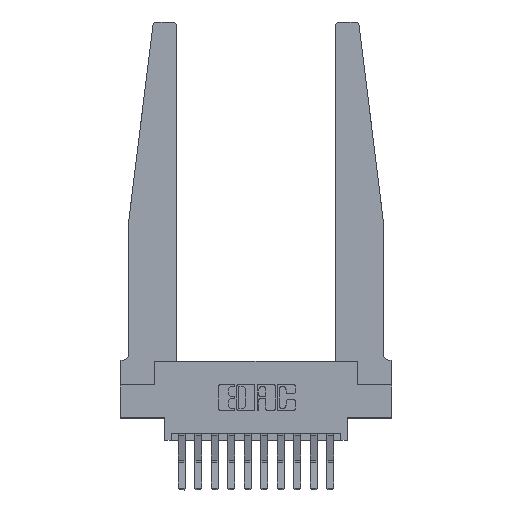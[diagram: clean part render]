
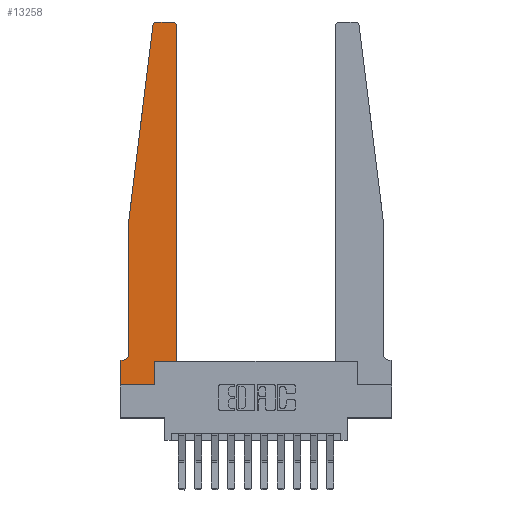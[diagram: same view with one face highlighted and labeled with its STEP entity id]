
A CAD part, top view. The second image highlights one B-rep face of the part: STEP entity #13258.
In plain terms, the highlighted planar face has unit normal (0, 0, 1).
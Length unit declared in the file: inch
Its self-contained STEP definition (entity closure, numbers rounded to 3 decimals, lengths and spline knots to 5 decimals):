
#75 = VERTEX_POINT ( 'NONE', #12826 ) ;
#86 = LINE ( 'NONE', #15667, #2582 ) ;
#128 = EDGE_CURVE ( 'NONE', #75, #3566, #86, .T. ) ;
#212 = DIRECTION ( 'NONE',  ( 0., 0., 1. ) ) ;
#662 = ORIENTED_EDGE ( 'NONE', *, *, #15537, .T. ) ;
#775 = AXIS2_PLACEMENT_3D ( 'NONE', #14170, #6856, #15410 ) ;
#1500 = LINE ( 'NONE', #12822, #10864 ) ;
#1690 = LINE ( 'NONE', #8300, #11048 ) ;
#1749 = EDGE_CURVE ( 'NONE', #13895, #6172, #13241, .T. ) ;
#2089 = EDGE_CURVE ( 'NONE', #12580, #13895, #5752, .T. ) ;
#2169 = DIRECTION ( 'NONE',  ( -0.122, -0.992, 0. ) ) ;
#2582 = VECTOR ( 'NONE', #8376, 39.37008 ) ;
#2801 = VERTEX_POINT ( 'NONE', #6228 ) ;
#3094 = VECTOR ( 'NONE', #2169, 39.37008 ) ;
#3345 = CARTESIAN_POINT ( 'NONE',  ( 0., 0.1875, 0.37 ) ) ;
#3473 = VECTOR ( 'NONE', #4188, 39.37008 ) ;
#3566 = VERTEX_POINT ( 'NONE', #9481 ) ;
#3702 = EDGE_CURVE ( 'NONE', #12538, #7731, #10699, .T. ) ;
#3711 = CARTESIAN_POINT ( 'NONE',  ( 0., 0.1875, 0.37 ) ) ;
#4159 = LINE ( 'NONE', #6285, #13909 ) ;
#4188 = DIRECTION ( 'NONE',  ( 1., 0., 0. ) ) ;
#4594 = DIRECTION ( 'NONE',  ( 0., 0., -1. ) ) ;
#4637 = DIRECTION ( 'NONE',  ( 0., -1., 0. ) ) ;
#4796 = CARTESIAN_POINT ( 'NONE',  ( 0., 0., 0.37 ) ) ;
#4827 = CARTESIAN_POINT ( 'NONE',  ( 0.2605, 0.18, 0.37 ) ) ;
#4869 = CARTESIAN_POINT ( 'NONE',  ( 0.425, 0.18, 0.37 ) ) ;
#5153 = EDGE_CURVE ( 'NONE', #2801, #8428, #14705, .T. ) ;
#5361 = CARTESIAN_POINT ( 'NONE',  ( 0.425, 0.18, 0.37 ) ) ;
#5443 = AXIS2_PLACEMENT_3D ( 'NONE', #3345, #7037, #15584 ) ;
#5482 = DIRECTION ( 'NONE',  ( -1., 0., 0. ) ) ;
#5547 = AXIS2_PLACEMENT_3D ( 'NONE', #7550, #212, #8792 ) ;
#5752 = LINE ( 'NONE', #4827, #11909 ) ;
#5829 = EDGE_LOOP ( 'NONE', ( #662, #6163, #9214, #6130, #12266, #8538, #13046, #6628, #7560, #15074, #10720, #9057 ) ) ;
#5873 = CARTESIAN_POINT ( 'NONE',  ( 0.015, 0.1875, 0.37 ) ) ;
#6130 = ORIENTED_EDGE ( 'NONE', *, *, #128, .T. ) ;
#6163 = ORIENTED_EDGE ( 'NONE', *, *, #3702, .T. ) ;
#6172 = VERTEX_POINT ( 'NONE', #4869 ) ;
#6228 = CARTESIAN_POINT ( 'NONE',  ( 0.425, 2.72, 0.37 ) ) ;
#6285 = CARTESIAN_POINT ( 'NONE',  ( 0., 0., 0.37 ) ) ;
#6332 = LINE ( 'NONE', #9475, #3094 ) ;
#6562 = CARTESIAN_POINT ( 'NONE',  ( 0.395, 2.75, 0.37 ) ) ;
#6628 = ORIENTED_EDGE ( 'NONE', *, *, #15398, .T. ) ;
#6856 = DIRECTION ( 'NONE',  ( 0., 0., 1. ) ) ;
#7037 = DIRECTION ( 'NONE',  ( 0., 0., 1. ) ) ;
#7222 = CARTESIAN_POINT ( 'NONE',  ( 0.065, 0.1875, 0.37 ) ) ;
#7550 = CARTESIAN_POINT ( 'NONE',  ( 0.27653, 2.72, 0.37 ) ) ;
#7560 = ORIENTED_EDGE ( 'NONE', *, *, #2089, .T. ) ;
#7731 = VERTEX_POINT ( 'NONE', #9168 ) ;
#8075 = EDGE_CURVE ( 'NONE', #12221, #10811, #9662, .T. ) ;
#8299 = DIRECTION ( 'NONE',  ( 0., 1., 0. ) ) ;
#8300 = CARTESIAN_POINT ( 'NONE',  ( 0., 0., 0.37 ) ) ;
#8320 = CIRCLE ( 'NONE', #14094, 0.05 ) ;
#8376 = DIRECTION ( 'NONE',  ( 0., -1., 0. ) ) ;
#8428 = VERTEX_POINT ( 'NONE', #6562 ) ;
#8532 = DIRECTION ( 'NONE',  ( 0., 1., 0. ) ) ;
#8538 = ORIENTED_EDGE ( 'NONE', *, *, #8075, .T. ) ;
#8792 = DIRECTION ( 'NONE',  ( 1., 0., 0. ) ) ;
#8852 = EDGE_CURVE ( 'NONE', #3566, #12221, #8320, .T. ) ;
#9057 = ORIENTED_EDGE ( 'NONE', *, *, #5153, .T. ) ;
#9106 = CARTESIAN_POINT ( 'NONE',  ( 0.27653, 2.75, 0.37 ) ) ;
#9168 = CARTESIAN_POINT ( 'NONE',  ( 0.24675, 2.72367, 0.37 ) ) ;
#9214 = ORIENTED_EDGE ( 'NONE', *, *, #9971, .T. ) ;
#9215 = CARTESIAN_POINT ( 'NONE',  ( 0.2605, 0., 0.37 ) ) ;
#9449 = CARTESIAN_POINT ( 'NONE',  ( 0.425, 0.18, 0.37 ) ) ;
#9475 = CARTESIAN_POINT ( 'NONE',  ( 0.065, 1.25, 0.37 ) ) ;
#9481 = CARTESIAN_POINT ( 'NONE',  ( 0.065, 0.2375, 0.37 ) ) ;
#9484 = CARTESIAN_POINT ( 'NONE',  ( 0.2605, 0.18, 0.37 ) ) ;
#9662 = LINE ( 'NONE', #7222, #15399 ) ;
#9685 = DIRECTION ( 'NONE',  ( -1., 0., 0. ) ) ;
#9971 = EDGE_CURVE ( 'NONE', #7731, #75, #6332, .T. ) ;
#10699 = CIRCLE ( 'NONE', #5547, 0.03 ) ;
#10720 = ORIENTED_EDGE ( 'NONE', *, *, #11621, .T. ) ;
#10805 = VERTEX_POINT ( 'NONE', #4796 ) ;
#10811 = VERTEX_POINT ( 'NONE', #3711 ) ;
#10864 = VECTOR ( 'NONE', #5482, 39.37008 ) ;
#11048 = VECTOR ( 'NONE', #4637, 39.37008 ) ;
#11112 = VECTOR ( 'NONE', #8299, 39.37008 ) ;
#11621 = EDGE_CURVE ( 'NONE', #6172, #2801, #14339, .T. ) ;
#11909 = VECTOR ( 'NONE', #8532, 39.37008 ) ;
#11927 = PLANE ( 'NONE',  #5443 ) ;
#11939 = CARTESIAN_POINT ( 'NONE',  ( 0.015, 0.2375, 0.37 ) ) ;
#12221 = VERTEX_POINT ( 'NONE', #5873 ) ;
#12266 = ORIENTED_EDGE ( 'NONE', *, *, #8852, .T. ) ;
#12538 = VERTEX_POINT ( 'NONE', #9106 ) ;
#12580 = VERTEX_POINT ( 'NONE', #9215 ) ;
#12822 = CARTESIAN_POINT ( 'NONE',  ( 0.25, 2.75, 0.37 ) ) ;
#12826 = CARTESIAN_POINT ( 'NONE',  ( 0.065, 1.25, 0.37 ) ) ;
#13046 = ORIENTED_EDGE ( 'NONE', *, *, #15746, .T. ) ;
#13147 = DIRECTION ( 'NONE',  ( -1., 0., 0. ) ) ;
#13241 = LINE ( 'NONE', #5361, #3473 ) ;
#13258 = ADVANCED_FACE ( 'NONE', ( #14521 ), #11927, .T. ) ;
#13619 = DIRECTION ( 'NONE',  ( 1., 0., 0. ) ) ;
#13895 = VERTEX_POINT ( 'NONE', #9484 ) ;
#13909 = VECTOR ( 'NONE', #13619, 39.37008 ) ;
#14094 = AXIS2_PLACEMENT_3D ( 'NONE', #11939, #4594, #13147 ) ;
#14170 = CARTESIAN_POINT ( 'NONE',  ( 0.395, 2.72, 0.37 ) ) ;
#14339 = LINE ( 'NONE', #9449, #11112 ) ;
#14521 = FACE_OUTER_BOUND ( 'NONE', #5829, .T. ) ;
#14705 = CIRCLE ( 'NONE', #775, 0.03 ) ;
#15074 = ORIENTED_EDGE ( 'NONE', *, *, #1749, .T. ) ;
#15398 = EDGE_CURVE ( 'NONE', #10805, #12580, #4159, .T. ) ;
#15399 = VECTOR ( 'NONE', #9685, 39.37008 ) ;
#15410 = DIRECTION ( 'NONE',  ( 1., 0., 0. ) ) ;
#15537 = EDGE_CURVE ( 'NONE', #8428, #12538, #1500, .T. ) ;
#15584 = DIRECTION ( 'NONE',  ( 1., 0., 0. ) ) ;
#15667 = CARTESIAN_POINT ( 'NONE',  ( 0.065, 1.25, 0.37 ) ) ;
#15746 = EDGE_CURVE ( 'NONE', #10811, #10805, #1690, .T. ) ;
